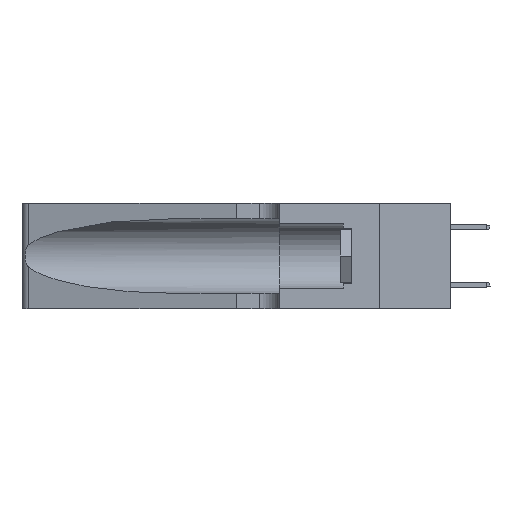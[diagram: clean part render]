
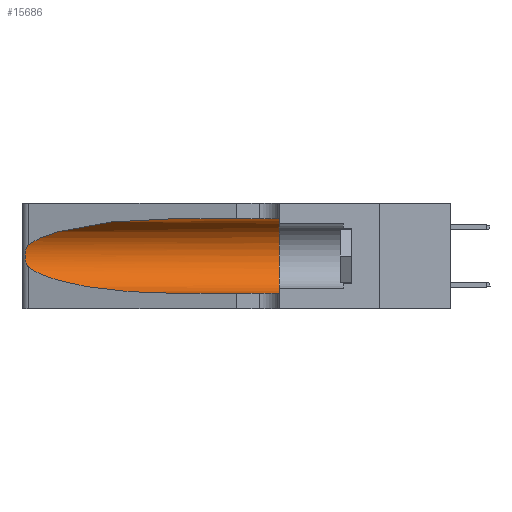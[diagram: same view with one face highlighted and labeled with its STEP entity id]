
A CAD part, left-side view. The second image highlights one B-rep face of the part: STEP entity #15686.
In plain terms, the highlighted cylindrical face has radius 3.308 mm (diameter 6.617 mm), a partial arc.
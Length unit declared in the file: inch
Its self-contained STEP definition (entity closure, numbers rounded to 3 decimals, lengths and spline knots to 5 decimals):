
#30 = EDGE_CURVE ( 'NONE', #15723, #2346, #2061, .T. ) ;
#273 = VECTOR ( 'NONE', #17612, 39.37008 ) ;
#574 = CARTESIAN_POINT ( 'NONE',  ( 0.25787, 1.23484, 0.2124 ) ) ;
#879 = CARTESIAN_POINT ( 'NONE',  ( 0.18966, 0.96281, 0.31525 ) ) ;
#1261 = CARTESIAN_POINT ( 'NONE',  ( 0.1305, 0.35, 0.185 ) ) ;
#1974 = CARTESIAN_POINT ( 'NONE',  ( 0.1305, 1.61858, 0.05475 ) ) ;
#2061 =( BOUNDED_CURVE ( )  B_SPLINE_CURVE ( 3, ( #6465, #10566, #17029, #21136 ),
 .UNSPECIFIED., .F., .T. ) 
 B_SPLINE_CURVE_WITH_KNOTS ( ( 4, 4 ),
 ( 3.44316, 4.71239 ),
 .UNSPECIFIED. ) 
 CURVE ( )  GEOMETRIC_REPRESENTATION_ITEM ( )  RATIONAL_B_SPLINE_CURVE ( ( 1., 0.87, 0.87, 1. ) ) 
 REPRESENTATION_ITEM ( '' )  );
#2346 = VERTEX_POINT ( 'NONE', #15774 ) ;
#3136 = CARTESIAN_POINT ( 'NONE',  ( 0.1305, 0.72297, 0.31525 ) ) ;
#3263 = DIRECTION ( 'NONE',  ( 0., 0., 1. ) ) ;
#3398 = CARTESIAN_POINT ( 'NONE',  ( 0.25487, 1.22718, 0.22369 ) ) ;
#3658 = CARTESIAN_POINT ( 'NONE',  ( 0.25487, 1.22718, 0.22369 ) ) ;
#4344 = CIRCLE ( 'NONE', #16603, 0.13025 ) ;
#4682 = CARTESIAN_POINT ( 'NONE',  ( 0.26017, 1.23833, 0.17102 ) ) ;
#5350 = CARTESIAN_POINT ( 'NONE',  ( 0.1305, 1.61858, 0.31525 ) ) ;
#5477 = LINE ( 'NONE', #5350, #19350 ) ;
#5508 = EDGE_CURVE ( 'NONE', #11407, #20871, #4344, .T. ) ;
#5527 = DIRECTION ( 'NONE',  ( 0., 0., -1. ) ) ;
#5948 = LINE ( 'NONE', #1974, #273 ) ;
#6144 = CARTESIAN_POINT ( 'NONE',  ( 0.1305, 0.72297, 0.31525 ) ) ;
#6465 = CARTESIAN_POINT ( 'NONE',  ( 0.25487, 1.22718, 0.14631 ) ) ;
#6546 = CARTESIAN_POINT ( 'NONE',  ( 0.25555, 1.22994, 0.2215 ) ) ;
#7199 = DIRECTION ( 'NONE',  ( 0., -1., 0. ) ) ;
#7471 = CARTESIAN_POINT ( 'NONE',  ( 0.1305, 0.35, 0.31525 ) ) ;
#7644 = CARTESIAN_POINT ( 'NONE',  ( 0.1305, 1.61858, 0.185 ) ) ;
#7776 = CYLINDRICAL_SURFACE ( 'NONE', #23237, 0.13025 ) ;
#8266 = ORIENTED_EDGE ( 'NONE', *, *, #5508, .F. ) ;
#8890 = EDGE_CURVE ( 'NONE', #19857, #9031, #22994, .T. ) ;
#9031 = VERTEX_POINT ( 'NONE', #3658 ) ;
#10109 = ORIENTED_EDGE ( 'NONE', *, *, #20001, .T. ) ;
#10386 = CARTESIAN_POINT ( 'NONE',  ( 0.25639, 1.23186, 0.15144 ) ) ;
#10566 = CARTESIAN_POINT ( 'NONE',  ( 0.2373, 1.15595, 0.08982 ) ) ;
#11408 = EDGE_CURVE ( 'NONE', #19857, #11407, #5477, .T. ) ;
#11407 = VERTEX_POINT ( 'NONE', #7471 ) ;
#11789 = ORIENTED_EDGE ( 'NONE', *, *, #11408, .F. ) ;
#12032 = EDGE_CURVE ( 'NONE', #2346, #20871, #5948, .T. ) ;
#12758 = CARTESIAN_POINT ( 'NONE',  ( 0.25856, 1.23593, 0.16098 ) ) ;
#13255 = EDGE_LOOP ( 'NONE', ( #25654, #10109, #25939, #21328, #8266, #11789 ) ) ;
#13316 = B_SPLINE_CURVE_WITH_KNOTS ( 'NONE', 3,
 ( #16863, #6546, #14606, #574, #14742, #18611, #14341, #22803, #4682, #12758, #22407, #10386, #24896, #20832 ),
 .UNSPECIFIED., .F., .F.,
 ( 4, 2, 2, 2, 2, 2, 4 ),
 ( 0., 0.00027, 0.00053, 0.00107, 0.0016, 0.00187, 0.00214 ),
 .UNSPECIFIED. ) ;
#13859 = CARTESIAN_POINT ( 'NONE',  ( 0.25487, 1.22718, 0.14631 ) ) ;
#14341 = CARTESIAN_POINT ( 'NONE',  ( 0.26075, 1.23896, 0.19203 ) ) ;
#14606 = CARTESIAN_POINT ( 'NONE',  ( 0.25639, 1.23184, 0.21858 ) ) ;
#14742 = CARTESIAN_POINT ( 'NONE',  ( 0.25854, 1.2359, 0.20912 ) ) ;
#15686 = ADVANCED_FACE ( 'NONE', ( #19830 ), #7776, .F. ) ;
#15723 = VERTEX_POINT ( 'NONE', #13859 ) ;
#15774 = CARTESIAN_POINT ( 'NONE',  ( 0.1305, 0.72297, 0.05475 ) ) ;
#16603 = AXIS2_PLACEMENT_3D ( 'NONE', #1261, #23215, #3263 ) ;
#16863 = CARTESIAN_POINT ( 'NONE',  ( 0.25487, 1.22718, 0.22369 ) ) ;
#17029 = CARTESIAN_POINT ( 'NONE',  ( 0.18966, 0.96281, 0.05475 ) ) ;
#17612 = DIRECTION ( 'NONE',  ( 0., -1., 0. ) ) ;
#18611 = CARTESIAN_POINT ( 'NONE',  ( 0.26018, 1.23835, 0.19895 ) ) ;
#19035 = CARTESIAN_POINT ( 'NONE',  ( 0.2373, 1.15595, 0.28018 ) ) ;
#19350 = VECTOR ( 'NONE', #7199, 39.37008 ) ;
#19830 = FACE_OUTER_BOUND ( 'NONE', #13255, .T. ) ;
#19857 = VERTEX_POINT ( 'NONE', #6144 ) ;
#20001 = EDGE_CURVE ( 'NONE', #9031, #15723, #13316, .T. ) ;
#20832 = CARTESIAN_POINT ( 'NONE',  ( 0.25487, 1.22718, 0.14631 ) ) ;
#20871 = VERTEX_POINT ( 'NONE', #21333 ) ;
#21136 = CARTESIAN_POINT ( 'NONE',  ( 0.1305, 0.72297, 0.05475 ) ) ;
#21328 = ORIENTED_EDGE ( 'NONE', *, *, #12032, .T. ) ;
#21333 = CARTESIAN_POINT ( 'NONE',  ( 0.1305, 0.35, 0.05475 ) ) ;
#22407 = CARTESIAN_POINT ( 'NONE',  ( 0.25789, 1.23486, 0.15765 ) ) ;
#22803 = CARTESIAN_POINT ( 'NONE',  ( 0.26075, 1.23896, 0.178 ) ) ;
#22994 =( BOUNDED_CURVE ( )  B_SPLINE_CURVE ( 3, ( #3136, #879, #19035, #3398 ),
 .UNSPECIFIED., .F., .T. ) 
 B_SPLINE_CURVE_WITH_KNOTS ( ( 4, 4 ),
 ( 1.5708, 2.84003 ),
 .UNSPECIFIED. ) 
 CURVE ( )  GEOMETRIC_REPRESENTATION_ITEM ( )  RATIONAL_B_SPLINE_CURVE ( ( 1., 0.87, 0.87, 1. ) ) 
 REPRESENTATION_ITEM ( '' )  );
#23215 = DIRECTION ( 'NONE',  ( 0., 1., 0. ) ) ;
#23237 = AXIS2_PLACEMENT_3D ( 'NONE', #7644, #23625, #5527 ) ;
#23625 = DIRECTION ( 'NONE',  ( 0., -1., 0. ) ) ;
#24896 = CARTESIAN_POINT ( 'NONE',  ( 0.25555, 1.22993, 0.14849 ) ) ;
#25654 = ORIENTED_EDGE ( 'NONE', *, *, #8890, .T. ) ;
#25939 = ORIENTED_EDGE ( 'NONE', *, *, #30, .T. ) ;
